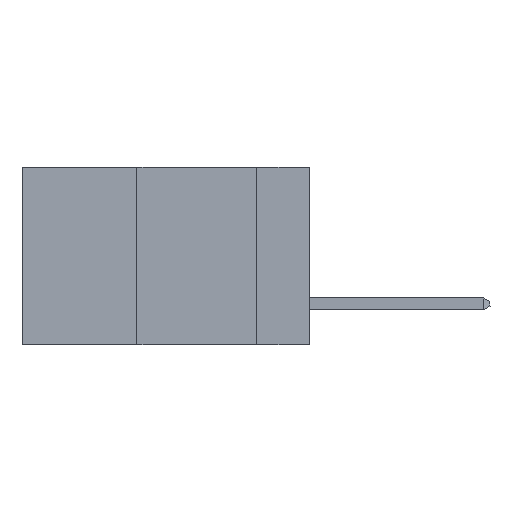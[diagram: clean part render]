
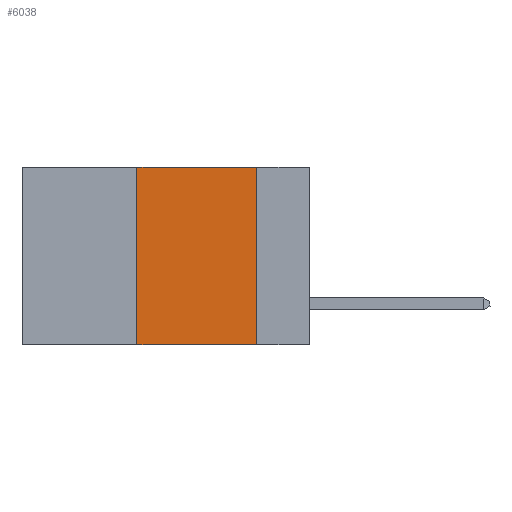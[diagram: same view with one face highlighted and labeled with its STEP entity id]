
A CAD part, left-side view. The second image highlights one B-rep face of the part: STEP entity #6038.
In plain terms, the highlighted planar face has unit normal (-1, 0, 0).
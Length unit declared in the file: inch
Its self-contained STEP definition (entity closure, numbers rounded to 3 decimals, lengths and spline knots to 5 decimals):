
#675 = EDGE_CURVE ( 'NONE', #7005, #805, #6621, .T. ) ;
#805 = VERTEX_POINT ( 'NONE', #6975 ) ;
#1907 = ORIENTED_EDGE ( 'NONE', *, *, #4600, .F. ) ;
#1959 = FACE_OUTER_BOUND ( 'NONE', #7083, .T. ) ;
#2229 = ORIENTED_EDGE ( 'NONE', *, *, #11790, .T. ) ;
#2723 = PLANE ( 'NONE',  #6267 ) ;
#2962 = DIRECTION ( 'NONE',  ( 0., -1., 0. ) ) ;
#3154 = LINE ( 'NONE', #12220, #3799 ) ;
#3799 = VECTOR ( 'NONE', #12619, 39.37008 ) ;
#4056 = VECTOR ( 'NONE', #6502, 39.37008 ) ;
#4329 = DIRECTION ( 'NONE',  ( 0., 0., -1. ) ) ;
#4475 = CARTESIAN_POINT ( 'NONE',  ( 0., 0.36, 0. ) ) ;
#4600 = EDGE_CURVE ( 'NONE', #10377, #7005, #3154, .T. ) ;
#5833 = DIRECTION ( 'NONE',  ( 0., 0., -1. ) ) ;
#5842 = LINE ( 'NONE', #8923, #10236 ) ;
#6038 = ADVANCED_FACE ( 'NONE', ( #1959 ), #2723, .F. ) ;
#6267 = AXIS2_PLACEMENT_3D ( 'NONE', #7844, #12283, #4329 ) ;
#6337 = VECTOR ( 'NONE', #5833, 39.37008 ) ;
#6502 = DIRECTION ( 'NONE',  ( 0., 0., 1. ) ) ;
#6621 = LINE ( 'NONE', #8763, #6337 ) ;
#6975 = CARTESIAN_POINT ( 'NONE',  ( 0., 0.11, -0.37 ) ) ;
#7005 = VERTEX_POINT ( 'NONE', #11891 ) ;
#7083 = EDGE_LOOP ( 'NONE', ( #11879, #1907, #7293, #2229 ) ) ;
#7293 = ORIENTED_EDGE ( 'NONE', *, *, #12098, .F. ) ;
#7822 = VERTEX_POINT ( 'NONE', #8215 ) ;
#7844 = CARTESIAN_POINT ( 'NONE',  ( 0., 0.6, 0. ) ) ;
#8215 = CARTESIAN_POINT ( 'NONE',  ( 0., 0.36, -0.37 ) ) ;
#8763 = CARTESIAN_POINT ( 'NONE',  ( 0., 0.11, 0. ) ) ;
#8923 = CARTESIAN_POINT ( 'NONE',  ( 0., 0.6, -0.37 ) ) ;
#9288 = LINE ( 'NONE', #9354, #4056 ) ;
#9354 = CARTESIAN_POINT ( 'NONE',  ( 0., 0.36, 0. ) ) ;
#10236 = VECTOR ( 'NONE', #2962, 39.37008 ) ;
#10377 = VERTEX_POINT ( 'NONE', #4475 ) ;
#11790 = EDGE_CURVE ( 'NONE', #7822, #805, #5842, .T. ) ;
#11879 = ORIENTED_EDGE ( 'NONE', *, *, #675, .F. ) ;
#11891 = CARTESIAN_POINT ( 'NONE',  ( 0., 0.11, 0. ) ) ;
#12098 = EDGE_CURVE ( 'NONE', #7822, #10377, #9288, .T. ) ;
#12220 = CARTESIAN_POINT ( 'NONE',  ( 0., 0.6, 0. ) ) ;
#12283 = DIRECTION ( 'NONE',  ( 1., 0., 0. ) ) ;
#12619 = DIRECTION ( 'NONE',  ( 0., -1., 0. ) ) ;
